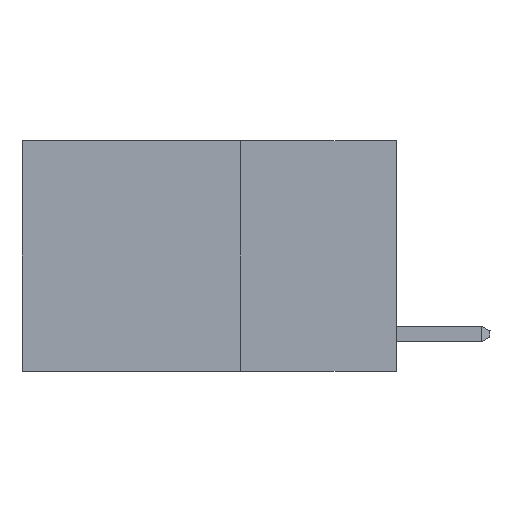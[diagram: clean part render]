
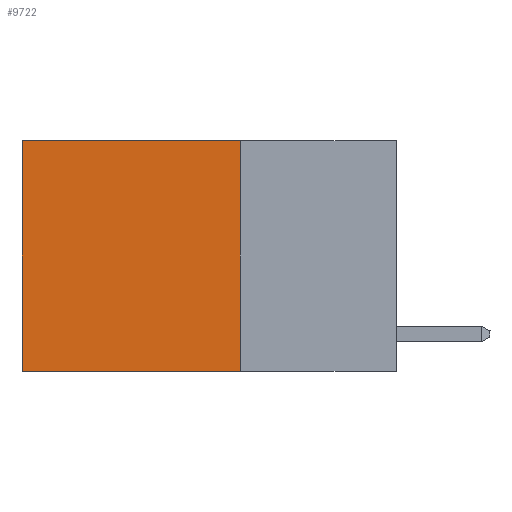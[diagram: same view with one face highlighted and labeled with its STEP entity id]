
A CAD part, left-side view. The second image highlights one B-rep face of the part: STEP entity #9722.
In plain terms, the highlighted planar face has unit normal (-1, 0, 0).
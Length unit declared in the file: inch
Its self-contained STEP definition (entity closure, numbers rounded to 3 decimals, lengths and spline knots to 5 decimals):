
#32 = CARTESIAN_POINT ( 'NONE',  ( 0.2625, 0.25, -0.37 ) ) ;
#146 = VERTEX_POINT ( 'NONE', #24813 ) ;
#266 = VERTEX_POINT ( 'NONE', #13460 ) ;
#480 = CARTESIAN_POINT ( 'NONE',  ( 0.2625, 0.6, 0. ) ) ;
#1257 = VECTOR ( 'NONE', #24855, 39.37008 ) ;
#2080 = DIRECTION ( 'NONE',  ( 0., 0., -1. ) ) ;
#2358 = EDGE_CURVE ( 'NONE', #8235, #266, #3414, .T. ) ;
#2727 = LINE ( 'NONE', #32, #1257 ) ;
#3414 = LINE ( 'NONE', #480, #6387 ) ;
#4056 = CARTESIAN_POINT ( 'NONE',  ( 0.2625, 0.25, 0. ) ) ;
#4734 = AXIS2_PLACEMENT_3D ( 'NONE', #19945, #21613, #18066 ) ;
#5480 = EDGE_CURVE ( 'NONE', #22031, #8235, #23738, .T. ) ;
#6387 = VECTOR ( 'NONE', #15898, 39.37008 ) ;
#6403 = PLANE ( 'NONE',  #4734 ) ;
#7354 = CARTESIAN_POINT ( 'NONE',  ( 0.2625, 0.25, 0. ) ) ;
#7361 = FACE_OUTER_BOUND ( 'NONE', #9748, .T. ) ;
#8115 = EDGE_CURVE ( 'NONE', #22031, #146, #14427, .T. ) ;
#8235 = VERTEX_POINT ( 'NONE', #14044 ) ;
#9557 = ORIENTED_EDGE ( 'NONE', *, *, #5480, .T. ) ;
#9722 = ADVANCED_FACE ( 'NONE', ( #7361 ), #6403, .F. ) ;
#9748 = EDGE_LOOP ( 'NONE', ( #15911, #19934, #17504, #9557 ) ) ;
#12664 = DIRECTION ( 'NONE',  ( 0., 1., 0. ) ) ;
#13460 = CARTESIAN_POINT ( 'NONE',  ( 0.2625, 0.6, -0.37 ) ) ;
#14044 = CARTESIAN_POINT ( 'NONE',  ( 0.2625, 0.6, 0. ) ) ;
#14427 = LINE ( 'NONE', #4056, #17433 ) ;
#15322 = VECTOR ( 'NONE', #12664, 39.37008 ) ;
#15898 = DIRECTION ( 'NONE',  ( 0., 0., -1. ) ) ;
#15911 = ORIENTED_EDGE ( 'NONE', *, *, #2358, .T. ) ;
#17433 = VECTOR ( 'NONE', #2080, 39.37008 ) ;
#17504 = ORIENTED_EDGE ( 'NONE', *, *, #8115, .F. ) ;
#18066 = DIRECTION ( 'NONE',  ( 0., 0., -1. ) ) ;
#19934 = ORIENTED_EDGE ( 'NONE', *, *, #24190, .F. ) ;
#19945 = CARTESIAN_POINT ( 'NONE',  ( 0.2625, 0.25, 0. ) ) ;
#21613 = DIRECTION ( 'NONE',  ( 1., 0., 0. ) ) ;
#22031 = VERTEX_POINT ( 'NONE', #7354 ) ;
#23738 = LINE ( 'NONE', #24204, #15322 ) ;
#24190 = EDGE_CURVE ( 'NONE', #146, #266, #2727, .T. ) ;
#24204 = CARTESIAN_POINT ( 'NONE',  ( 0.2625, 0.25, 0. ) ) ;
#24813 = CARTESIAN_POINT ( 'NONE',  ( 0.2625, 0.25, -0.37 ) ) ;
#24855 = DIRECTION ( 'NONE',  ( 0., 1., 0. ) ) ;
